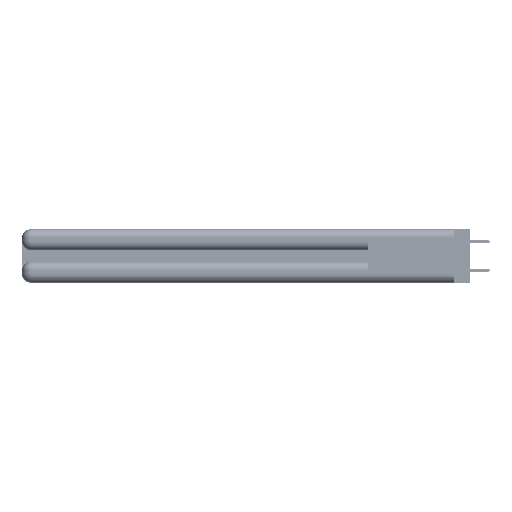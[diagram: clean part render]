
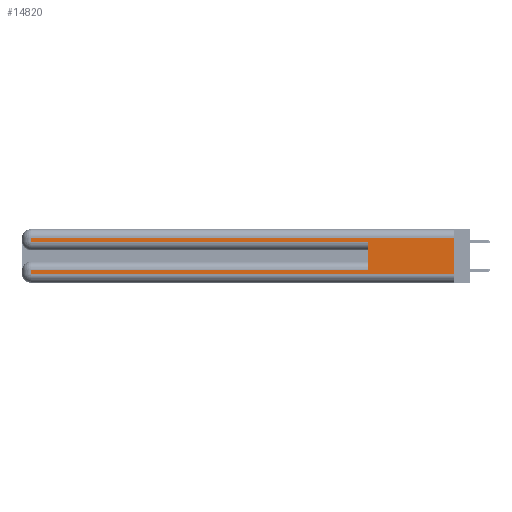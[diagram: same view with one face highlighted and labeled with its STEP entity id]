
A CAD part, left-side view. The second image highlights one B-rep face of the part: STEP entity #14820.
In plain terms, the highlighted planar face has unit normal (-1, 0, 0).
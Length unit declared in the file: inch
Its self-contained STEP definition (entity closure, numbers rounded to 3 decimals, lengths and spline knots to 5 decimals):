
#135 = EDGE_CURVE ( 'NONE', #20187, #47925, #45649, .T. ) ;
#1046 = DIRECTION ( 'NONE',  ( 0., 1., 0. ) ) ;
#1212 = DIRECTION ( 'NONE',  ( 0., 0., -1. ) ) ;
#1776 = DIRECTION ( 'NONE',  ( 1., 0., 0. ) ) ;
#6911 = CARTESIAN_POINT ( 'NONE',  ( 0., 0., 0.285 ) ) ;
#7215 = LINE ( 'NONE', #51759, #18046 ) ;
#7360 = DIRECTION ( 'NONE',  ( 0., 0., -1. ) ) ;
#7371 = EDGE_LOOP ( 'NONE', ( #30771, #9874, #46211, #7950, #45733, #29790, #31371, #46042 ) ) ;
#7784 = CARTESIAN_POINT ( 'NONE',  ( 0., 2.94, 0.285 ) ) ;
#7950 = ORIENTED_EDGE ( 'NONE', *, *, #135, .T. ) ;
#8709 = EDGE_CURVE ( 'NONE', #41557, #50910, #42737, .T. ) ;
#9874 = ORIENTED_EDGE ( 'NONE', *, *, #8709, .T. ) ;
#10143 = VECTOR ( 'NONE', #48684, 39.37008 ) ;
#10513 = EDGE_CURVE ( 'NONE', #32411, #47925, #42547, .T. ) ;
#10732 = CARTESIAN_POINT ( 'NONE',  ( 0., 2.94, 0.37 ) ) ;
#11413 = VERTEX_POINT ( 'NONE', #25490 ) ;
#13153 = CARTESIAN_POINT ( 'NONE',  ( 0., 0., 0.31 ) ) ;
#13537 = VERTEX_POINT ( 'NONE', #51486 ) ;
#14796 = VECTOR ( 'NONE', #43215, 39.37008 ) ;
#14820 = ADVANCED_FACE ( 'NONE', ( #48370 ), #21994, .F. ) ;
#16214 = CARTESIAN_POINT ( 'NONE',  ( 0., 0.6, 0.145 ) ) ;
#18046 = VECTOR ( 'NONE', #27416, 39.37008 ) ;
#18765 = CARTESIAN_POINT ( 'NONE',  ( 0., 0.6, 0.285 ) ) ;
#20187 = VERTEX_POINT ( 'NONE', #7784 ) ;
#20768 = AXIS2_PLACEMENT_3D ( 'NONE', #26088, #1776, #30196 ) ;
#21961 = EDGE_CURVE ( 'NONE', #13537, #48624, #7215, .T. ) ;
#21994 = PLANE ( 'NONE',  #20768 ) ;
#23294 = CARTESIAN_POINT ( 'NONE',  ( 0., 0., 0.06 ) ) ;
#23992 = VECTOR ( 'NONE', #51297, 39.37008 ) ;
#25320 = EDGE_CURVE ( 'NONE', #11413, #13537, #46275, .T. ) ;
#25490 = CARTESIAN_POINT ( 'NONE',  ( 0., 2.94, 0.085 ) ) ;
#25569 = EDGE_CURVE ( 'NONE', #32411, #11413, #44336, .T. ) ;
#26088 = CARTESIAN_POINT ( 'NONE',  ( 0., 0., 0.37 ) ) ;
#26887 = EDGE_CURVE ( 'NONE', #50910, #20187, #47181, .T. ) ;
#27416 = DIRECTION ( 'NONE',  ( 0., -1., 0. ) ) ;
#29790 = ORIENTED_EDGE ( 'NONE', *, *, #25569, .T. ) ;
#30196 = DIRECTION ( 'NONE',  ( 0., 0., -1. ) ) ;
#30771 = ORIENTED_EDGE ( 'NONE', *, *, #46377, .F. ) ;
#31371 = ORIENTED_EDGE ( 'NONE', *, *, #25320, .T. ) ;
#31738 = CARTESIAN_POINT ( 'NONE',  ( 0., 0., 0.37 ) ) ;
#32411 = VERTEX_POINT ( 'NONE', #41832 ) ;
#34837 = VECTOR ( 'NONE', #43525, 39.37008 ) ;
#39029 = CARTESIAN_POINT ( 'NONE',  ( 0., 0., 0.085 ) ) ;
#40195 = VECTOR ( 'NONE', #1046, 39.37008 ) ;
#41557 = VERTEX_POINT ( 'NONE', #45168 ) ;
#41832 = CARTESIAN_POINT ( 'NONE',  ( 0., 0.6, 0.085 ) ) ;
#42547 = LINE ( 'NONE', #16214, #10143 ) ;
#42642 = CARTESIAN_POINT ( 'NONE',  ( 0., 2.94, 0.31 ) ) ;
#42737 = LINE ( 'NONE', #13153, #40195 ) ;
#43215 = DIRECTION ( 'NONE',  ( 0., 0., -1. ) ) ;
#43525 = DIRECTION ( 'NONE',  ( 0., -1., 0. ) ) ;
#44336 = LINE ( 'NONE', #39029, #23992 ) ;
#44999 = VECTOR ( 'NONE', #1212, 39.37008 ) ;
#45168 = CARTESIAN_POINT ( 'NONE',  ( 0., 0., 0.31 ) ) ;
#45407 = LINE ( 'NONE', #31738, #52398 ) ;
#45649 = LINE ( 'NONE', #6911, #34837 ) ;
#45733 = ORIENTED_EDGE ( 'NONE', *, *, #10513, .F. ) ;
#46042 = ORIENTED_EDGE ( 'NONE', *, *, #21961, .T. ) ;
#46211 = ORIENTED_EDGE ( 'NONE', *, *, #26887, .T. ) ;
#46275 = LINE ( 'NONE', #49883, #44999 ) ;
#46377 = EDGE_CURVE ( 'NONE', #41557, #48624, #45407, .T. ) ;
#47181 = LINE ( 'NONE', #10732, #14796 ) ;
#47925 = VERTEX_POINT ( 'NONE', #18765 ) ;
#48370 = FACE_OUTER_BOUND ( 'NONE', #7371, .T. ) ;
#48624 = VERTEX_POINT ( 'NONE', #23294 ) ;
#48684 = DIRECTION ( 'NONE',  ( 0., 0., 1. ) ) ;
#49883 = CARTESIAN_POINT ( 'NONE',  ( 0., 2.94, 0.37 ) ) ;
#50910 = VERTEX_POINT ( 'NONE', #42642 ) ;
#51297 = DIRECTION ( 'NONE',  ( 0., 1., 0. ) ) ;
#51486 = CARTESIAN_POINT ( 'NONE',  ( 0., 2.94, 0.06 ) ) ;
#51759 = CARTESIAN_POINT ( 'NONE',  ( 0., 0., 0.06 ) ) ;
#52398 = VECTOR ( 'NONE', #7360, 39.37008 ) ;
